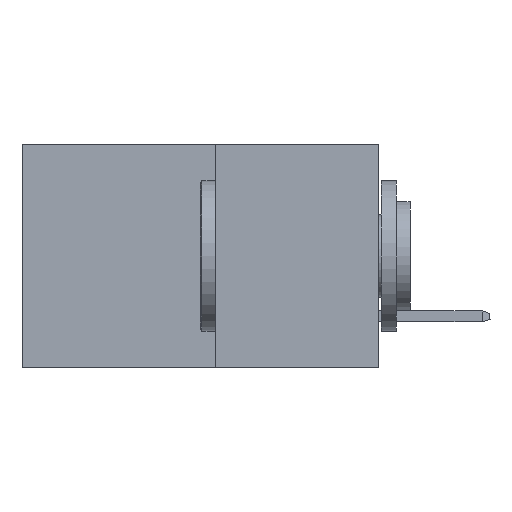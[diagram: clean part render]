
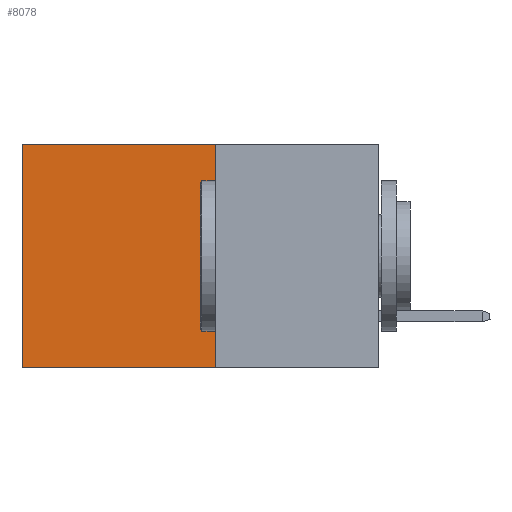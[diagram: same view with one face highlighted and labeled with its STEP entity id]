
A CAD part, left-side view. The second image highlights one B-rep face of the part: STEP entity #8078.
In plain terms, the highlighted planar face has unit normal (-1, 0, 0).
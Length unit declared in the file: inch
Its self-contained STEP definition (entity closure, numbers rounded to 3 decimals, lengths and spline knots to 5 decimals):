
#900 = CARTESIAN_POINT ( 'NONE',  ( 0.277, 0.27, 0. ) ) ;
#1535 = DIRECTION ( 'NONE',  ( 0., 1., 0. ) ) ;
#2452 = ORIENTED_EDGE ( 'NONE', *, *, #17288, .T. ) ;
#3037 = CARTESIAN_POINT ( 'NONE',  ( 0.277, 0.27, -0.37 ) ) ;
#3243 = EDGE_CURVE ( 'NONE', #4792, #5320, #15333, .T. ) ;
#3252 = EDGE_LOOP ( 'NONE', ( #4803, #8815, #16436, #2452 ) ) ;
#3313 = PLANE ( 'NONE',  #10674 ) ;
#3619 = CARTESIAN_POINT ( 'NONE',  ( 0.277, 0.59, -0.37 ) ) ;
#4232 = VECTOR ( 'NONE', #15834, 39.37008 ) ;
#4767 = VECTOR ( 'NONE', #9220, 39.37008 ) ;
#4792 = VERTEX_POINT ( 'NONE', #9712 ) ;
#4803 = ORIENTED_EDGE ( 'NONE', *, *, #11578, .T. ) ;
#5320 = VERTEX_POINT ( 'NONE', #3619 ) ;
#5992 = CARTESIAN_POINT ( 'NONE',  ( 0.277, 0.27, 0. ) ) ;
#6064 = DIRECTION ( 'NONE',  ( 1., 0., 0. ) ) ;
#7110 = DIRECTION ( 'NONE',  ( 0., 0., -1. ) ) ;
#8078 = ADVANCED_FACE ( 'NONE', ( #8171 ), #3313, .F. ) ;
#8171 = FACE_OUTER_BOUND ( 'NONE', #3252, .T. ) ;
#8815 = ORIENTED_EDGE ( 'NONE', *, *, #3243, .F. ) ;
#9220 = DIRECTION ( 'NONE',  ( 0., 0., -1. ) ) ;
#9712 = CARTESIAN_POINT ( 'NONE',  ( 0.277, 0.27, -0.37 ) ) ;
#10674 = AXIS2_PLACEMENT_3D ( 'NONE', #14170, #6064, #15528 ) ;
#11250 = VECTOR ( 'NONE', #7110, 39.37008 ) ;
#11428 = LINE ( 'NONE', #900, #4232 ) ;
#11578 = EDGE_CURVE ( 'NONE', #16166, #5320, #15577, .T. ) ;
#11699 = VECTOR ( 'NONE', #1535, 39.37008 ) ;
#12405 = VERTEX_POINT ( 'NONE', #5992 ) ;
#12490 = CARTESIAN_POINT ( 'NONE',  ( 0.277, 0.59, 0. ) ) ;
#14170 = CARTESIAN_POINT ( 'NONE',  ( 0.277, 0.27, -0.37 ) ) ;
#14208 = CARTESIAN_POINT ( 'NONE',  ( 0.277, 0.27, -0.37 ) ) ;
#15315 = LINE ( 'NONE', #3037, #11250 ) ;
#15333 = LINE ( 'NONE', #14208, #11699 ) ;
#15528 = DIRECTION ( 'NONE',  ( 0., 0., -1. ) ) ;
#15577 = LINE ( 'NONE', #15977, #4767 ) ;
#15834 = DIRECTION ( 'NONE',  ( 0., 1., 0. ) ) ;
#15977 = CARTESIAN_POINT ( 'NONE',  ( 0.277, 0.59, -0.37 ) ) ;
#16166 = VERTEX_POINT ( 'NONE', #12490 ) ;
#16168 = EDGE_CURVE ( 'NONE', #12405, #4792, #15315, .T. ) ;
#16436 = ORIENTED_EDGE ( 'NONE', *, *, #16168, .F. ) ;
#17288 = EDGE_CURVE ( 'NONE', #12405, #16166, #11428, .T. ) ;
